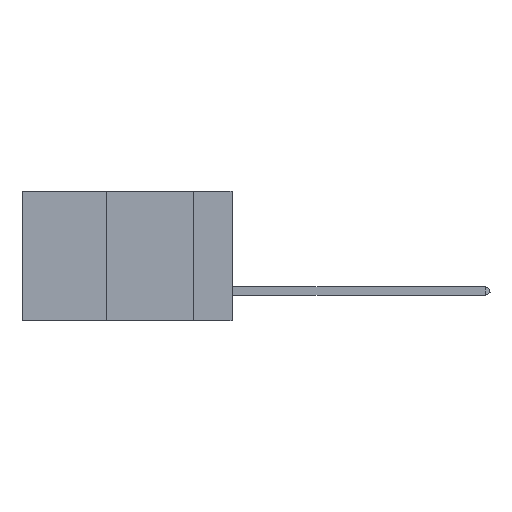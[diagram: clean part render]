
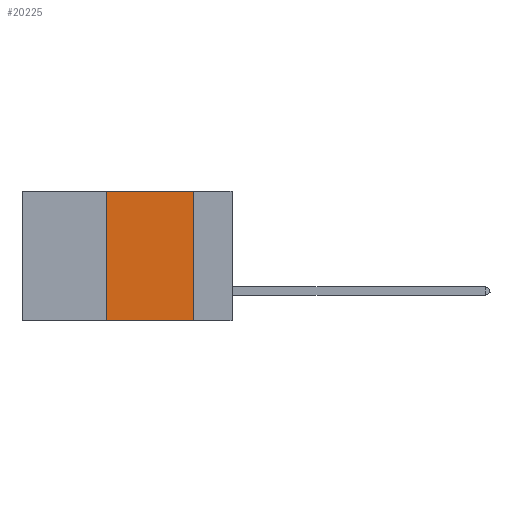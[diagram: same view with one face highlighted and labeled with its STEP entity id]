
A CAD part, left-side view. The second image highlights one B-rep face of the part: STEP entity #20225.
In plain terms, the highlighted planar face has unit normal (-1, 0, 0).
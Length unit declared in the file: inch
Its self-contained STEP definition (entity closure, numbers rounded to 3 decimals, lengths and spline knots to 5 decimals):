
#615 = CARTESIAN_POINT ( 'NONE',  ( 0., 0.11, 0. ) ) ;
#1639 = CARTESIAN_POINT ( 'NONE',  ( 0., 0.6, 0. ) ) ;
#4221 = PLANE ( 'NONE',  #7600 ) ;
#4569 = DIRECTION ( 'NONE',  ( 0., 0., -1. ) ) ;
#5972 = ORIENTED_EDGE ( 'NONE', *, *, #19680, .F. ) ;
#7600 = AXIS2_PLACEMENT_3D ( 'NONE', #1639, #29825, #4569 ) ;
#9000 = EDGE_CURVE ( 'NONE', #17090, #21762, #18844, .T. ) ;
#10182 = CARTESIAN_POINT ( 'NONE',  ( 0., 0.36, 0. ) ) ;
#10459 = CARTESIAN_POINT ( 'NONE',  ( 0., 0.36, 0. ) ) ;
#12321 = DIRECTION ( 'NONE',  ( 0., 0., -1. ) ) ;
#12839 = ORIENTED_EDGE ( 'NONE', *, *, #26229, .F. ) ;
#12955 = DIRECTION ( 'NONE',  ( 0., -1., 0. ) ) ;
#13022 = CARTESIAN_POINT ( 'NONE',  ( 0., 0.11, -0.37 ) ) ;
#13116 = DIRECTION ( 'NONE',  ( 0., 0., 1. ) ) ;
#14337 = LINE ( 'NONE', #10459, #24322 ) ;
#16086 = VECTOR ( 'NONE', #12955, 39.37008 ) ;
#16187 = CARTESIAN_POINT ( 'NONE',  ( 0., 0.36, -0.37 ) ) ;
#16319 = VERTEX_POINT ( 'NONE', #615 ) ;
#17090 = VERTEX_POINT ( 'NONE', #16187 ) ;
#18799 = ORIENTED_EDGE ( 'NONE', *, *, #9000, .T. ) ;
#18844 = LINE ( 'NONE', #30779, #16086 ) ;
#19680 = EDGE_CURVE ( 'NONE', #25047, #16319, #30316, .T. ) ;
#19849 = FACE_OUTER_BOUND ( 'NONE', #20062, .T. ) ;
#20062 = EDGE_LOOP ( 'NONE', ( #12839, #5972, #29625, #18799 ) ) ;
#20225 = ADVANCED_FACE ( 'NONE', ( #19849 ), #4221, .F. ) ;
#21762 = VERTEX_POINT ( 'NONE', #13022 ) ;
#21910 = VECTOR ( 'NONE', #12321, 39.37008 ) ;
#24322 = VECTOR ( 'NONE', #13116, 39.37008 ) ;
#24615 = EDGE_CURVE ( 'NONE', #17090, #25047, #14337, .T. ) ;
#25047 = VERTEX_POINT ( 'NONE', #10182 ) ;
#26035 = DIRECTION ( 'NONE',  ( 0., -1., 0. ) ) ;
#26229 = EDGE_CURVE ( 'NONE', #16319, #21762, #32224, .T. ) ;
#27937 = VECTOR ( 'NONE', #26035, 39.37008 ) ;
#29625 = ORIENTED_EDGE ( 'NONE', *, *, #24615, .F. ) ;
#29825 = DIRECTION ( 'NONE',  ( 1., 0., 0. ) ) ;
#30316 = LINE ( 'NONE', #30805, #27937 ) ;
#30779 = CARTESIAN_POINT ( 'NONE',  ( 0., 0.6, -0.37 ) ) ;
#30805 = CARTESIAN_POINT ( 'NONE',  ( 0., 0.6, 0. ) ) ;
#32224 = LINE ( 'NONE', #32243, #21910 ) ;
#32243 = CARTESIAN_POINT ( 'NONE',  ( 0., 0.11, 0. ) ) ;
